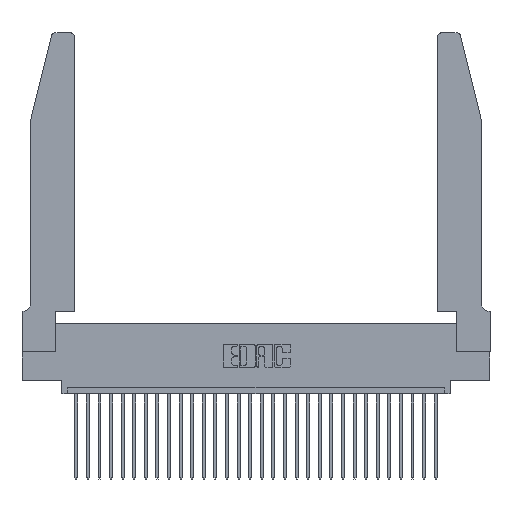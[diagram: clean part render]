
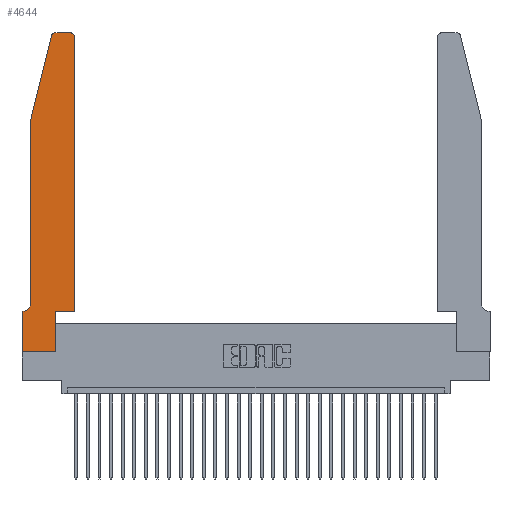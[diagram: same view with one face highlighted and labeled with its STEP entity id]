
A CAD part, top view. The second image highlights one B-rep face of the part: STEP entity #4644.
In plain terms, the highlighted planar face has unit normal (0, 0, 1).
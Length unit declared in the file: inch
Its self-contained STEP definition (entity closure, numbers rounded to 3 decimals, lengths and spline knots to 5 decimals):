
#103 = LINE ( 'NONE', #6501, #12903 ) ;
#473 = AXIS2_PLACEMENT_3D ( 'NONE', #23212, #27956, #501 ) ;
#498 = CARTESIAN_POINT ( 'NONE',  ( 0.0055, 0.35, 0.37 ) ) ;
#501 = DIRECTION ( 'NONE',  ( 1., 0., 0. ) ) ;
#1138 = CIRCLE ( 'NONE', #473, 0.03 ) ;
#1213 = DIRECTION ( 'NONE',  ( -1., 0., 0. ) ) ;
#1647 = VERTEX_POINT ( 'NONE', #28200 ) ;
#2233 = VERTEX_POINT ( 'NONE', #18180 ) ;
#3755 = DIRECTION ( 'NONE',  ( 0., -1., 0. ) ) ;
#4150 = VERTEX_POINT ( 'NONE', #8087 ) ;
#4312 = EDGE_CURVE ( 'NONE', #21976, #7311, #15613, .T. ) ;
#4481 = CARTESIAN_POINT ( 'NONE',  ( 0.4505, 0.35, 0.37 ) ) ;
#4644 = ADVANCED_FACE ( 'NONE', ( #7549 ), #27250, .T. ) ;
#4652 = CARTESIAN_POINT ( 'NONE',  ( 0.4505, 0.35, 0.37 ) ) ;
#4783 = LINE ( 'NONE', #18657, #7335 ) ;
#4848 = CIRCLE ( 'NONE', #24895, 0.07 ) ;
#5263 = VECTOR ( 'NONE', #28531, 39.37008 ) ;
#5303 = CARTESIAN_POINT ( 'NONE',  ( 0.2865, 0.35, 0.37 ) ) ;
#5395 = ORIENTED_EDGE ( 'NONE', *, *, #14993, .T. ) ;
#5482 = VERTEX_POINT ( 'NONE', #23165 ) ;
#5510 = VECTOR ( 'NONE', #3755, 39.37008 ) ;
#5656 = EDGE_CURVE ( 'NONE', #1647, #20291, #6347, .T. ) ;
#5813 = EDGE_LOOP ( 'NONE', ( #26905, #14600, #17380, #11660, #25993, #27230, #14681, #9754, #15498, #19167, #5395, #25846 ) ) ;
#5900 = DIRECTION ( 'NONE',  ( 1., 0., 0. ) ) ;
#6329 = EDGE_CURVE ( 'NONE', #20291, #21976, #4848, .T. ) ;
#6347 = LINE ( 'NONE', #16476, #5263 ) ;
#6361 = EDGE_CURVE ( 'NONE', #17701, #12725, #103, .T. ) ;
#6501 = CARTESIAN_POINT ( 'NONE',  ( 0.2605, 2.75, 0.37 ) ) ;
#6910 = CARTESIAN_POINT ( 'NONE',  ( 0.0755, 0.35, 0.37 ) ) ;
#7311 = VERTEX_POINT ( 'NONE', #27439 ) ;
#7335 = VECTOR ( 'NONE', #18849, 39.37008 ) ;
#7403 = LINE ( 'NONE', #5303, #29741 ) ;
#7549 = FACE_OUTER_BOUND ( 'NONE', #5813, .T. ) ;
#7723 = EDGE_CURVE ( 'NONE', #8151, #15048, #7403, .T. ) ;
#8087 = CARTESIAN_POINT ( 'NONE',  ( 0.4505, 2.72, 0.37 ) ) ;
#8151 = VERTEX_POINT ( 'NONE', #8431 ) ;
#8431 = CARTESIAN_POINT ( 'NONE',  ( 0.2865, 0., 0.37 ) ) ;
#8526 = EDGE_CURVE ( 'NONE', #2233, #8151, #24601, .T. ) ;
#8598 = DIRECTION ( 'NONE',  ( 0., 0., 1. ) ) ;
#8646 = DIRECTION ( 'NONE',  ( 0., 1., 0. ) ) ;
#9339 = DIRECTION ( 'NONE',  ( 1., 0., 0. ) ) ;
#9389 = EDGE_CURVE ( 'NONE', #12725, #5482, #1138, .T. ) ;
#9754 = ORIENTED_EDGE ( 'NONE', *, *, #8526, .T. ) ;
#9818 = VECTOR ( 'NONE', #8646, 39.37008 ) ;
#10308 = LINE ( 'NONE', #4652, #24263 ) ;
#11551 = AXIS2_PLACEMENT_3D ( 'NONE', #28655, #26152, #23887 ) ;
#11660 = ORIENTED_EDGE ( 'NONE', *, *, #5656, .T. ) ;
#12688 = AXIS2_PLACEMENT_3D ( 'NONE', #13423, #8598, #13134 ) ;
#12725 = VERTEX_POINT ( 'NONE', #24324 ) ;
#12903 = VECTOR ( 'NONE', #18445, 39.37008 ) ;
#13134 = DIRECTION ( 'NONE',  ( 1., 0., 0. ) ) ;
#13423 = CARTESIAN_POINT ( 'NONE',  ( 0., 0.35, 0.37 ) ) ;
#14146 = VECTOR ( 'NONE', #30252, 39.37008 ) ;
#14286 = LINE ( 'NONE', #22670, #5510 ) ;
#14600 = ORIENTED_EDGE ( 'NONE', *, *, #9389, .T. ) ;
#14681 = ORIENTED_EDGE ( 'NONE', *, *, #26520, .T. ) ;
#14993 = EDGE_CURVE ( 'NONE', #15564, #4150, #22305, .T. ) ;
#15048 = VERTEX_POINT ( 'NONE', #27831 ) ;
#15185 = DIRECTION ( 'NONE',  ( 0., 0., -1. ) ) ;
#15498 = ORIENTED_EDGE ( 'NONE', *, *, #7723, .T. ) ;
#15564 = VERTEX_POINT ( 'NONE', #20357 ) ;
#15613 = LINE ( 'NONE', #6910, #14146 ) ;
#16476 = CARTESIAN_POINT ( 'NONE',  ( 0.0755, 2., 0.37 ) ) ;
#16833 = DIRECTION ( 'NONE',  ( 0., 1., 0. ) ) ;
#16991 = CIRCLE ( 'NONE', #11551, 0.03 ) ;
#17380 = ORIENTED_EDGE ( 'NONE', *, *, #26742, .T. ) ;
#17701 = VERTEX_POINT ( 'NONE', #26660 ) ;
#18065 = EDGE_CURVE ( 'NONE', #15048, #15564, #10308, .T. ) ;
#18180 = CARTESIAN_POINT ( 'NONE',  ( 0., 0., 0.37 ) ) ;
#18445 = DIRECTION ( 'NONE',  ( -1., 0., 0. ) ) ;
#18657 = CARTESIAN_POINT ( 'NONE',  ( 0.0755, 2., 0.37 ) ) ;
#18849 = DIRECTION ( 'NONE',  ( -0.239, -0.971, 0. ) ) ;
#19167 = ORIENTED_EDGE ( 'NONE', *, *, #18065, .T. ) ;
#20207 = CARTESIAN_POINT ( 'NONE',  ( 0., 0., 0.37 ) ) ;
#20291 = VERTEX_POINT ( 'NONE', #25396 ) ;
#20357 = CARTESIAN_POINT ( 'NONE',  ( 0.4505, 0.35, 0.37 ) ) ;
#21976 = VERTEX_POINT ( 'NONE', #498 ) ;
#22305 = LINE ( 'NONE', #4481, #9818 ) ;
#22670 = CARTESIAN_POINT ( 'NONE',  ( 0., 0., 0.37 ) ) ;
#23165 = CARTESIAN_POINT ( 'NONE',  ( 0.25487, 2.72718, 0.37 ) ) ;
#23212 = CARTESIAN_POINT ( 'NONE',  ( 0.284, 2.72, 0.37 ) ) ;
#23887 = DIRECTION ( 'NONE',  ( 1., 0., 0. ) ) ;
#24263 = VECTOR ( 'NONE', #9339, 39.37008 ) ;
#24324 = CARTESIAN_POINT ( 'NONE',  ( 0.284, 2.75, 0.37 ) ) ;
#24601 = LINE ( 'NONE', #20207, #29002 ) ;
#24895 = AXIS2_PLACEMENT_3D ( 'NONE', #25023, #15185, #1213 ) ;
#25023 = CARTESIAN_POINT ( 'NONE',  ( 0.0055, 0.42, 0.37 ) ) ;
#25396 = CARTESIAN_POINT ( 'NONE',  ( 0.0755, 0.42, 0.37 ) ) ;
#25846 = ORIENTED_EDGE ( 'NONE', *, *, #29475, .T. ) ;
#25993 = ORIENTED_EDGE ( 'NONE', *, *, #6329, .T. ) ;
#26152 = DIRECTION ( 'NONE',  ( 0., 0., 1. ) ) ;
#26520 = EDGE_CURVE ( 'NONE', #7311, #2233, #14286, .T. ) ;
#26660 = CARTESIAN_POINT ( 'NONE',  ( 0.4205, 2.75, 0.37 ) ) ;
#26742 = EDGE_CURVE ( 'NONE', #5482, #1647, #4783, .T. ) ;
#26905 = ORIENTED_EDGE ( 'NONE', *, *, #6361, .T. ) ;
#27230 = ORIENTED_EDGE ( 'NONE', *, *, #4312, .T. ) ;
#27250 = PLANE ( 'NONE',  #12688 ) ;
#27439 = CARTESIAN_POINT ( 'NONE',  ( 0., 0.35, 0.37 ) ) ;
#27831 = CARTESIAN_POINT ( 'NONE',  ( 0.2865, 0.35, 0.37 ) ) ;
#27956 = DIRECTION ( 'NONE',  ( 0., 0., 1. ) ) ;
#28200 = CARTESIAN_POINT ( 'NONE',  ( 0.0755, 2., 0.37 ) ) ;
#28531 = DIRECTION ( 'NONE',  ( 0., -1., 0. ) ) ;
#28655 = CARTESIAN_POINT ( 'NONE',  ( 0.4205, 2.72, 0.37 ) ) ;
#29002 = VECTOR ( 'NONE', #5900, 39.37008 ) ;
#29475 = EDGE_CURVE ( 'NONE', #4150, #17701, #16991, .T. ) ;
#29741 = VECTOR ( 'NONE', #16833, 39.37008 ) ;
#30252 = DIRECTION ( 'NONE',  ( -1., 0., 0. ) ) ;
